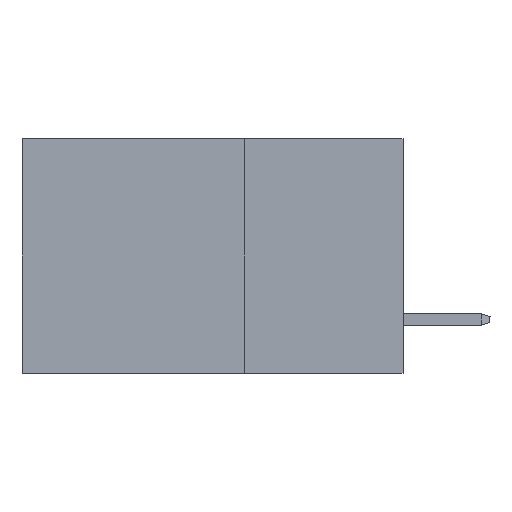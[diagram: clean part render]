
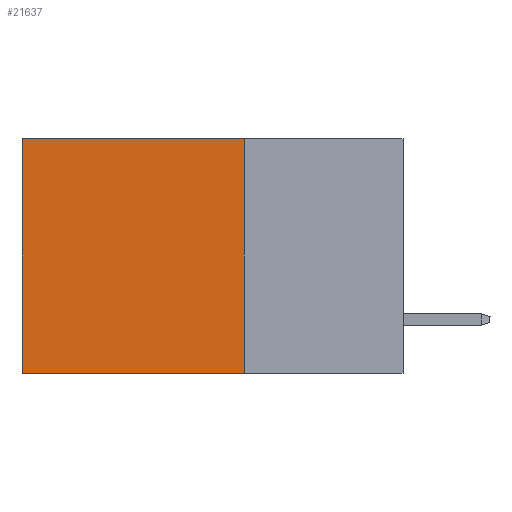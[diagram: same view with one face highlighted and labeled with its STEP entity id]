
A CAD part, left-side view. The second image highlights one B-rep face of the part: STEP entity #21637.
In plain terms, the highlighted planar face has unit normal (-1, 0, 0).
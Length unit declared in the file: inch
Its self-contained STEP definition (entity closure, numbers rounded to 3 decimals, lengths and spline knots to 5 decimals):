
#2125 = DIRECTION ( 'NONE',  ( 0., 0., -1. ) ) ;
#2558 = LINE ( 'NONE', #2808, #33431 ) ;
#2808 = CARTESIAN_POINT ( 'NONE',  ( 0.2875, 0.25, 0. ) ) ;
#3153 = CARTESIAN_POINT ( 'NONE',  ( 0.2875, 0.25, -0.37 ) ) ;
#3209 = EDGE_LOOP ( 'NONE', ( #8536, #13531, #25212, #36429 ) ) ;
#3298 = DIRECTION ( 'NONE',  ( 0., 0., -1. ) ) ;
#6939 = DIRECTION ( 'NONE',  ( 0., 1., 0. ) ) ;
#8536 = ORIENTED_EDGE ( 'NONE', *, *, #46964, .T. ) ;
#8762 = CARTESIAN_POINT ( 'NONE',  ( 0.2875, 0.6, -0.37 ) ) ;
#9256 = AXIS2_PLACEMENT_3D ( 'NONE', #27240, #23375, #15173 ) ;
#9791 = VERTEX_POINT ( 'NONE', #36062 ) ;
#11252 = LINE ( 'NONE', #46692, #46423 ) ;
#13531 = ORIENTED_EDGE ( 'NONE', *, *, #42679, .F. ) ;
#15173 = DIRECTION ( 'NONE',  ( 0., 0., -1. ) ) ;
#20023 = VERTEX_POINT ( 'NONE', #3153 ) ;
#21637 = ADVANCED_FACE ( 'NONE', ( #50422 ), #34969, .F. ) ;
#23375 = DIRECTION ( 'NONE',  ( 1., 0., 0. ) ) ;
#25212 = ORIENTED_EDGE ( 'NONE', *, *, #34725, .F. ) ;
#26689 = EDGE_CURVE ( 'NONE', #33249, #9791, #2558, .T. ) ;
#27240 = CARTESIAN_POINT ( 'NONE',  ( 0.2875, 0.25, 0. ) ) ;
#28847 = VECTOR ( 'NONE', #6939, 39.37008 ) ;
#29347 = CARTESIAN_POINT ( 'NONE',  ( 0.2875, 0.6, 0. ) ) ;
#29830 = CARTESIAN_POINT ( 'NONE',  ( 0.2875, 0.25, -0.37 ) ) ;
#30772 = CARTESIAN_POINT ( 'NONE',  ( 0.2875, 0.25, 0. ) ) ;
#33249 = VERTEX_POINT ( 'NONE', #30772 ) ;
#33431 = VECTOR ( 'NONE', #34156, 39.37008 ) ;
#34156 = DIRECTION ( 'NONE',  ( 0., 1., 0. ) ) ;
#34238 = LINE ( 'NONE', #29347, #47250 ) ;
#34725 = EDGE_CURVE ( 'NONE', #33249, #20023, #11252, .T. ) ;
#34969 = PLANE ( 'NONE',  #9256 ) ;
#36062 = CARTESIAN_POINT ( 'NONE',  ( 0.2875, 0.6, 0. ) ) ;
#36429 = ORIENTED_EDGE ( 'NONE', *, *, #26689, .T. ) ;
#42679 = EDGE_CURVE ( 'NONE', #20023, #50468, #49624, .T. ) ;
#46423 = VECTOR ( 'NONE', #3298, 39.37008 ) ;
#46692 = CARTESIAN_POINT ( 'NONE',  ( 0.2875, 0.25, 0. ) ) ;
#46964 = EDGE_CURVE ( 'NONE', #9791, #50468, #34238, .T. ) ;
#47250 = VECTOR ( 'NONE', #2125, 39.37008 ) ;
#49624 = LINE ( 'NONE', #29830, #28847 ) ;
#50422 = FACE_OUTER_BOUND ( 'NONE', #3209, .T. ) ;
#50468 = VERTEX_POINT ( 'NONE', #8762 ) ;
